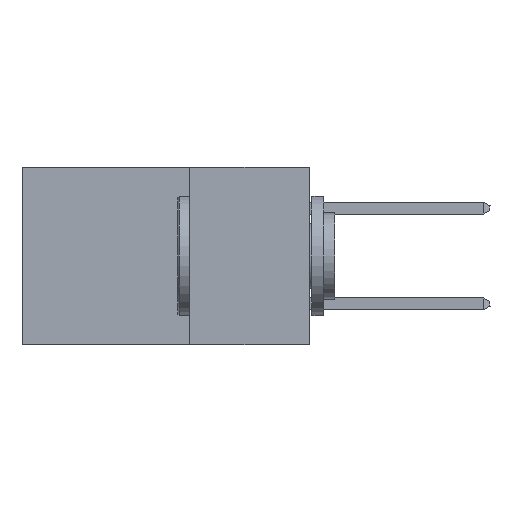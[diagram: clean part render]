
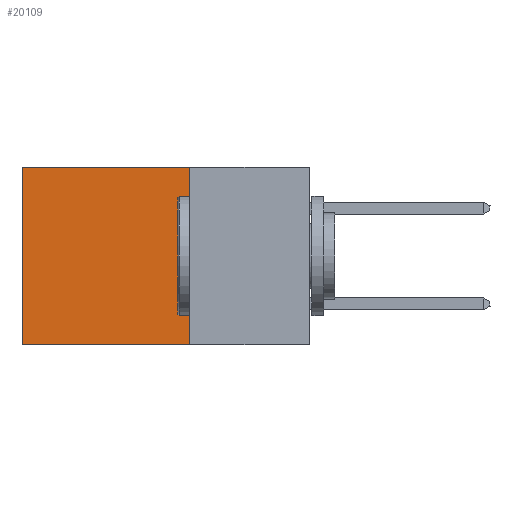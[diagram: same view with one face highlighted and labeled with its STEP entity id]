
A CAD part, left-side view. The second image highlights one B-rep face of the part: STEP entity #20109.
In plain terms, the highlighted planar face has unit normal (-1, 0, 0).
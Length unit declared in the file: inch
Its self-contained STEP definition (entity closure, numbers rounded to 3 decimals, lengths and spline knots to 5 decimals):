
#637 = CARTESIAN_POINT ( 'NONE',  ( 0.2875, 0.25, -0.37 ) ) ;
#996 = LINE ( 'NONE', #35863, #15036 ) ;
#1095 = LINE ( 'NONE', #35133, #19632 ) ;
#3378 = LINE ( 'NONE', #21470, #33798 ) ;
#4884 = EDGE_CURVE ( 'NONE', #43710, #27257, #996, .T. ) ;
#5141 = ORIENTED_EDGE ( 'NONE', *, *, #4884, .F. ) ;
#8542 = DIRECTION ( 'NONE',  ( 1., 0., 0. ) ) ;
#11475 = EDGE_CURVE ( 'NONE', #43710, #18484, #1095, .T. ) ;
#12335 = CARTESIAN_POINT ( 'NONE',  ( 0.2875, 0.25, 0. ) ) ;
#12903 = VERTEX_POINT ( 'NONE', #17668 ) ;
#14411 = CARTESIAN_POINT ( 'NONE',  ( 0.2875, 0.25, 0. ) ) ;
#15036 = VECTOR ( 'NONE', #39661, 39.37008 ) ;
#15478 = DIRECTION ( 'NONE',  ( 0., 0., -1. ) ) ;
#17484 = DIRECTION ( 'NONE',  ( 0., 1., 0. ) ) ;
#17668 = CARTESIAN_POINT ( 'NONE',  ( 0.2875, 0.6, -0.37 ) ) ;
#17895 = ORIENTED_EDGE ( 'NONE', *, *, #11475, .T. ) ;
#18347 = VECTOR ( 'NONE', #22151, 39.37008 ) ;
#18484 = VERTEX_POINT ( 'NONE', #24990 ) ;
#19632 = VECTOR ( 'NONE', #17484, 39.37008 ) ;
#20109 = ADVANCED_FACE ( 'NONE', ( #22675 ), #44795, .F. ) ;
#21470 = CARTESIAN_POINT ( 'NONE',  ( 0.2875, 0.6, 0. ) ) ;
#22151 = DIRECTION ( 'NONE',  ( 0., 1., 0. ) ) ;
#22675 = FACE_OUTER_BOUND ( 'NONE', #23020, .T. ) ;
#23020 = EDGE_LOOP ( 'NONE', ( #42298, #42330, #5141, #17895 ) ) ;
#24990 = CARTESIAN_POINT ( 'NONE',  ( 0.2875, 0.6, 0. ) ) ;
#27257 = VERTEX_POINT ( 'NONE', #34098 ) ;
#33798 = VECTOR ( 'NONE', #39146, 39.37008 ) ;
#34098 = CARTESIAN_POINT ( 'NONE',  ( 0.2875, 0.25, -0.37 ) ) ;
#35133 = CARTESIAN_POINT ( 'NONE',  ( 0.2875, 0.25, 0. ) ) ;
#35863 = CARTESIAN_POINT ( 'NONE',  ( 0.2875, 0.25, 0. ) ) ;
#36660 = EDGE_CURVE ( 'NONE', #27257, #12903, #36975, .T. ) ;
#36975 = LINE ( 'NONE', #637, #18347 ) ;
#39146 = DIRECTION ( 'NONE',  ( 0., 0., -1. ) ) ;
#39661 = DIRECTION ( 'NONE',  ( 0., 0., -1. ) ) ;
#40106 = EDGE_CURVE ( 'NONE', #18484, #12903, #3378, .T. ) ;
#40685 = AXIS2_PLACEMENT_3D ( 'NONE', #12335, #8542, #15478 ) ;
#42298 = ORIENTED_EDGE ( 'NONE', *, *, #40106, .T. ) ;
#42330 = ORIENTED_EDGE ( 'NONE', *, *, #36660, .F. ) ;
#43710 = VERTEX_POINT ( 'NONE', #14411 ) ;
#44795 = PLANE ( 'NONE',  #40685 ) ;
